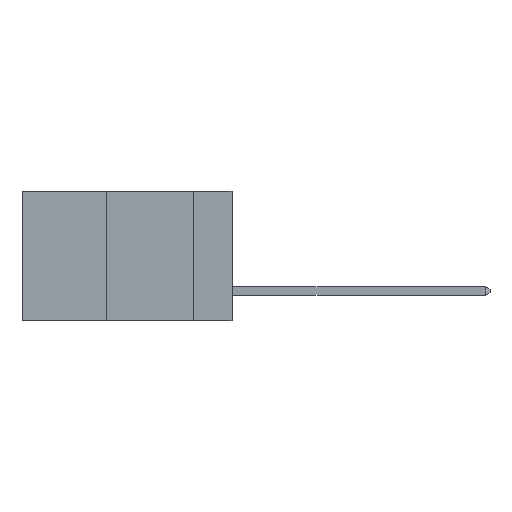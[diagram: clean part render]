
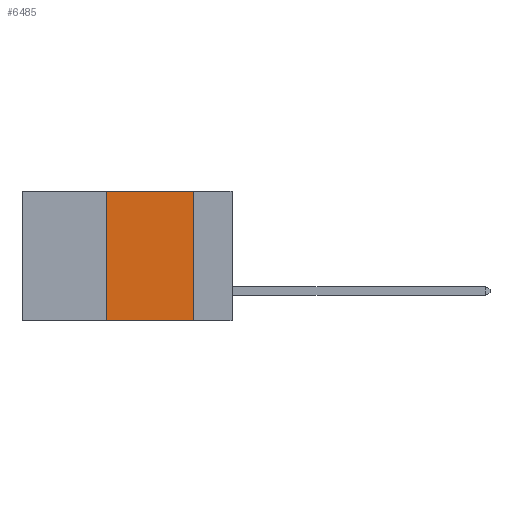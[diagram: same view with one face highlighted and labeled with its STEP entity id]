
A CAD part, left-side view. The second image highlights one B-rep face of the part: STEP entity #6485.
In plain terms, the highlighted planar face has unit normal (-1, 0, 0).
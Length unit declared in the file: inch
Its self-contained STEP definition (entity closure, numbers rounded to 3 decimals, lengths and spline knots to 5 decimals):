
#1175 = CARTESIAN_POINT ( 'NONE',  ( 0., 0.6, -0.37 ) ) ;
#1314 = LINE ( 'NONE', #8530, #12985 ) ;
#1348 = CARTESIAN_POINT ( 'NONE',  ( 0., 0.36, -0.37 ) ) ;
#2034 = VECTOR ( 'NONE', #11037, 39.37008 ) ;
#2618 = CARTESIAN_POINT ( 'NONE',  ( 0., 0.11, -0.37 ) ) ;
#3625 = PLANE ( 'NONE',  #12428 ) ;
#3876 = LINE ( 'NONE', #1175, #10044 ) ;
#4159 = VERTEX_POINT ( 'NONE', #2618 ) ;
#4832 = DIRECTION ( 'NONE',  ( 0., 0., -1. ) ) ;
#5783 = ORIENTED_EDGE ( 'NONE', *, *, #12686, .F. ) ;
#5914 = VECTOR ( 'NONE', #11840, 39.37008 ) ;
#6165 = ORIENTED_EDGE ( 'NONE', *, *, #6565, .T. ) ;
#6294 = LINE ( 'NONE', #7529, #5914 ) ;
#6485 = ADVANCED_FACE ( 'NONE', ( #10720 ), #3625, .F. ) ;
#6507 = CARTESIAN_POINT ( 'NONE',  ( 0., 0.11, 0. ) ) ;
#6565 = EDGE_CURVE ( 'NONE', #8713, #4159, #3876, .T. ) ;
#7127 = CARTESIAN_POINT ( 'NONE',  ( 0., 0.6, 0. ) ) ;
#7372 = EDGE_CURVE ( 'NONE', #8713, #12434, #6294, .T. ) ;
#7529 = CARTESIAN_POINT ( 'NONE',  ( 0., 0.36, 0. ) ) ;
#8159 = EDGE_CURVE ( 'NONE', #10496, #4159, #14216, .T. ) ;
#8530 = CARTESIAN_POINT ( 'NONE',  ( 0., 0.6, 0. ) ) ;
#8713 = VERTEX_POINT ( 'NONE', #1348 ) ;
#9282 = CARTESIAN_POINT ( 'NONE',  ( 0., 0.11, 0. ) ) ;
#10044 = VECTOR ( 'NONE', #11763, 39.37008 ) ;
#10496 = VERTEX_POINT ( 'NONE', #9282 ) ;
#10720 = FACE_OUTER_BOUND ( 'NONE', #11074, .T. ) ;
#11037 = DIRECTION ( 'NONE',  ( 0., 0., -1. ) ) ;
#11074 = EDGE_LOOP ( 'NONE', ( #13962, #5783, #14628, #6165 ) ) ;
#11640 = DIRECTION ( 'NONE',  ( 1., 0., 0. ) ) ;
#11763 = DIRECTION ( 'NONE',  ( 0., -1., 0. ) ) ;
#11840 = DIRECTION ( 'NONE',  ( 0., 0., 1. ) ) ;
#12428 = AXIS2_PLACEMENT_3D ( 'NONE', #7127, #11640, #4832 ) ;
#12434 = VERTEX_POINT ( 'NONE', #14584 ) ;
#12686 = EDGE_CURVE ( 'NONE', #12434, #10496, #1314, .T. ) ;
#12985 = VECTOR ( 'NONE', #14986, 39.37008 ) ;
#13962 = ORIENTED_EDGE ( 'NONE', *, *, #8159, .F. ) ;
#14216 = LINE ( 'NONE', #6507, #2034 ) ;
#14584 = CARTESIAN_POINT ( 'NONE',  ( 0., 0.36, 0. ) ) ;
#14628 = ORIENTED_EDGE ( 'NONE', *, *, #7372, .F. ) ;
#14986 = DIRECTION ( 'NONE',  ( 0., -1., 0. ) ) ;
